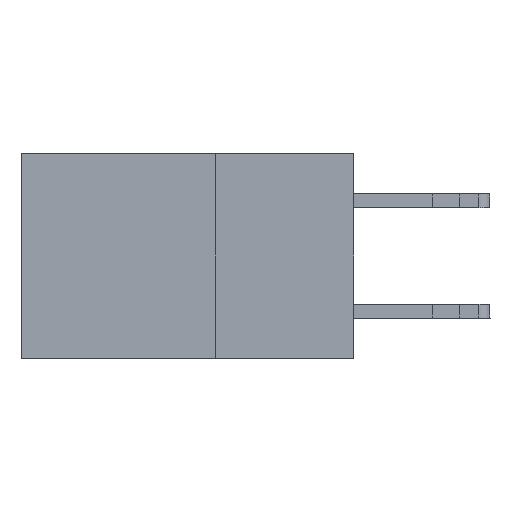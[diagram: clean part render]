
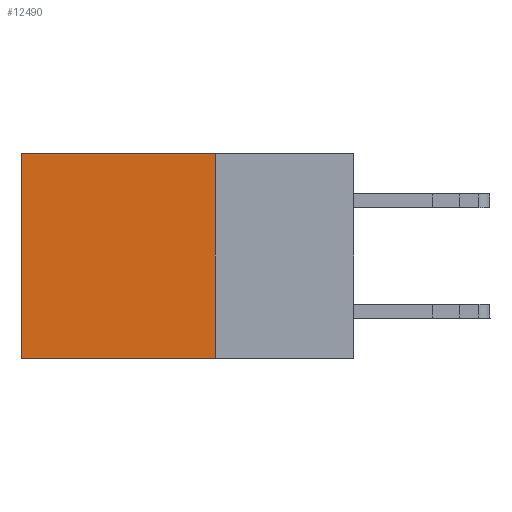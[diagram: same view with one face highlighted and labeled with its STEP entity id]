
A CAD part, left-side view. The second image highlights one B-rep face of the part: STEP entity #12490.
In plain terms, the highlighted planar face has unit normal (-1, 0, 0).
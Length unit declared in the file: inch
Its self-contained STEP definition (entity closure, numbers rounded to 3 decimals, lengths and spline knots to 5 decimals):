
#995 = PLANE ( 'NONE',  #27015 ) ;
#1018 = CARTESIAN_POINT ( 'NONE',  ( 0.2875, 0.6, 0. ) ) ;
#1147 = CARTESIAN_POINT ( 'NONE',  ( 0.2875, 0.6, 0. ) ) ;
#1948 = CARTESIAN_POINT ( 'NONE',  ( 0.2875, 0.25, -0.37 ) ) ;
#2225 = EDGE_CURVE ( 'NONE', #15205, #8084, #9002, .T. ) ;
#3177 = DIRECTION ( 'NONE',  ( 1., 0., 0. ) ) ;
#4711 = CARTESIAN_POINT ( 'NONE',  ( 0.2875, 0.25, 0. ) ) ;
#5451 = DIRECTION ( 'NONE',  ( 0., 0., -1. ) ) ;
#7741 = DIRECTION ( 'NONE',  ( 0., 0., -1. ) ) ;
#8084 = VERTEX_POINT ( 'NONE', #1948 ) ;
#8261 = EDGE_CURVE ( 'NONE', #21603, #14570, #18924, .T. ) ;
#8316 = VECTOR ( 'NONE', #21843, 39.37008 ) ;
#9002 = LINE ( 'NONE', #23022, #22289 ) ;
#12490 = ADVANCED_FACE ( 'NONE', ( #21328 ), #995, .F. ) ;
#12532 = LINE ( 'NONE', #15319, #8316 ) ;
#14030 = VECTOR ( 'NONE', #7741, 39.37008 ) ;
#14293 = CARTESIAN_POINT ( 'NONE',  ( 0.2875, 0.25, 0. ) ) ;
#14570 = VERTEX_POINT ( 'NONE', #17445 ) ;
#15205 = VERTEX_POINT ( 'NONE', #4711 ) ;
#15319 = CARTESIAN_POINT ( 'NONE',  ( 0.2875, 0.25, 0. ) ) ;
#15533 = LINE ( 'NONE', #23582, #25604 ) ;
#16792 = DIRECTION ( 'NONE',  ( 0., 1., 0. ) ) ;
#17445 = CARTESIAN_POINT ( 'NONE',  ( 0.2875, 0.6, -0.37 ) ) ;
#17814 = EDGE_LOOP ( 'NONE', ( #19887, #21906, #26993, #21593 ) ) ;
#18924 = LINE ( 'NONE', #1018, #14030 ) ;
#19245 = EDGE_CURVE ( 'NONE', #15205, #21603, #12532, .T. ) ;
#19887 = ORIENTED_EDGE ( 'NONE', *, *, #8261, .T. ) ;
#20713 = DIRECTION ( 'NONE',  ( 0., 0., -1. ) ) ;
#21328 = FACE_OUTER_BOUND ( 'NONE', #17814, .T. ) ;
#21593 = ORIENTED_EDGE ( 'NONE', *, *, #19245, .T. ) ;
#21603 = VERTEX_POINT ( 'NONE', #1147 ) ;
#21843 = DIRECTION ( 'NONE',  ( 0., 1., 0. ) ) ;
#21906 = ORIENTED_EDGE ( 'NONE', *, *, #28225, .F. ) ;
#22289 = VECTOR ( 'NONE', #20713, 39.37008 ) ;
#23022 = CARTESIAN_POINT ( 'NONE',  ( 0.2875, 0.25, 0. ) ) ;
#23582 = CARTESIAN_POINT ( 'NONE',  ( 0.2875, 0.25, -0.37 ) ) ;
#25604 = VECTOR ( 'NONE', #16792, 39.37008 ) ;
#26993 = ORIENTED_EDGE ( 'NONE', *, *, #2225, .F. ) ;
#27015 = AXIS2_PLACEMENT_3D ( 'NONE', #14293, #3177, #5451 ) ;
#28225 = EDGE_CURVE ( 'NONE', #8084, #14570, #15533, .T. ) ;
